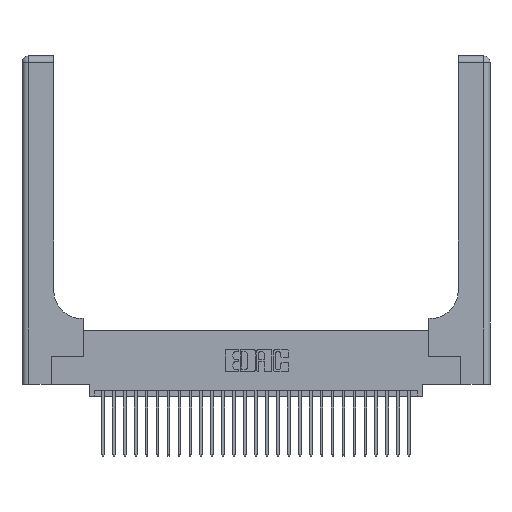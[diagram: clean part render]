
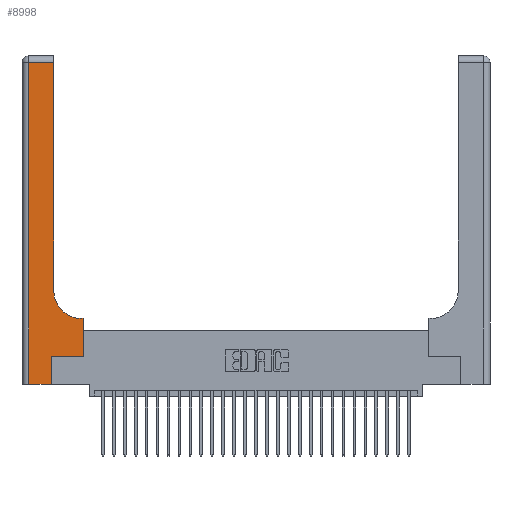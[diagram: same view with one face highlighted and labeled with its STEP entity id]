
A CAD part, top view. The second image highlights one B-rep face of the part: STEP entity #8998.
In plain terms, the highlighted planar face has unit normal (0, 0, 1).
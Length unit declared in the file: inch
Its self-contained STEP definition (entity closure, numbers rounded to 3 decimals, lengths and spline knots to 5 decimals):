
#754 = EDGE_CURVE ( 'NONE', #13265, #20896, #26308, .T. ) ;
#1070 = CIRCLE ( 'NONE', #4278, 0.25 ) ;
#1675 = EDGE_CURVE ( 'NONE', #7780, #22664, #6212, .T. ) ;
#1995 = CARTESIAN_POINT ( 'NONE',  ( 0., 2.94, 0.37 ) ) ;
#3305 = CARTESIAN_POINT ( 'NONE',  ( 0.5585, 0.25, 0.37 ) ) ;
#3576 = VERTEX_POINT ( 'NONE', #15224 ) ;
#3621 = DIRECTION ( 'NONE',  ( 0., 0., -1. ) ) ;
#3798 = CARTESIAN_POINT ( 'NONE',  ( 0.269, 0.25, 0.37 ) ) ;
#3932 = CARTESIAN_POINT ( 'NONE',  ( 0.5585, 0.6, 0.37 ) ) ;
#4256 = ORIENTED_EDGE ( 'NONE', *, *, #15265, .T. ) ;
#4278 = AXIS2_PLACEMENT_3D ( 'NONE', #15434, #3621, #26717 ) ;
#4520 = ORIENTED_EDGE ( 'NONE', *, *, #28610, .T. ) ;
#4866 = CARTESIAN_POINT ( 'NONE',  ( 0., 0., 0.37 ) ) ;
#5934 = DIRECTION ( 'NONE',  ( 1., 0., 0. ) ) ;
#6010 = FACE_OUTER_BOUND ( 'NONE', #8364, .T. ) ;
#6212 = LINE ( 'NONE', #3305, #18464 ) ;
#6389 = DIRECTION ( 'NONE',  ( 0., -1., 0. ) ) ;
#6430 = LINE ( 'NONE', #4866, #6605 ) ;
#6605 = VECTOR ( 'NONE', #23003, 39.37008 ) ;
#6891 = PLANE ( 'NONE',  #25453 ) ;
#6987 = CARTESIAN_POINT ( 'NONE',  ( 0., 3., 0.37 ) ) ;
#7747 = ORIENTED_EDGE ( 'NONE', *, *, #21952, .T. ) ;
#7780 = VERTEX_POINT ( 'NONE', #9403 ) ;
#8282 = VECTOR ( 'NONE', #20850, 39.37008 ) ;
#8323 = ORIENTED_EDGE ( 'NONE', *, *, #13071, .T. ) ;
#8364 = EDGE_LOOP ( 'NONE', ( #8323, #23698, #21033, #4256, #4520, #16832, #18394, #7747, #14993 ) ) ;
#8381 = LINE ( 'NONE', #16897, #18466 ) ;
#8575 = VERTEX_POINT ( 'NONE', #25861 ) ;
#8998 = ADVANCED_FACE ( 'NONE', ( #6010 ), #6891, .F. ) ;
#9403 = CARTESIAN_POINT ( 'NONE',  ( 0.5585, 0.25, 0.37 ) ) ;
#9794 = LINE ( 'NONE', #24581, #23461 ) ;
#11615 = CARTESIAN_POINT ( 'NONE',  ( 0.269, 0., 0.37 ) ) ;
#11818 = VERTEX_POINT ( 'NONE', #25079 ) ;
#12091 = DIRECTION ( 'NONE',  ( -1., 0., 0. ) ) ;
#12625 = LINE ( 'NONE', #11615, #8282 ) ;
#13071 = EDGE_CURVE ( 'NONE', #29853, #13265, #13387, .T. ) ;
#13265 = VERTEX_POINT ( 'NONE', #22595 ) ;
#13387 = LINE ( 'NONE', #17493, #26680 ) ;
#13688 = CARTESIAN_POINT ( 'NONE',  ( 0.269, 0.25, 0.37 ) ) ;
#14337 = EDGE_CURVE ( 'NONE', #16971, #7780, #27714, .T. ) ;
#14993 = ORIENTED_EDGE ( 'NONE', *, *, #22571, .T. ) ;
#15101 = CARTESIAN_POINT ( 'NONE',  ( 0.06, 2.94, 0.37 ) ) ;
#15103 = VECTOR ( 'NONE', #5934, 39.37008 ) ;
#15224 = CARTESIAN_POINT ( 'NONE',  ( 0.5415, 0.6, 0.37 ) ) ;
#15254 = CARTESIAN_POINT ( 'NONE',  ( 0.2915, 0.85, 0.37 ) ) ;
#15265 = EDGE_CURVE ( 'NONE', #8575, #11818, #6430, .T. ) ;
#15434 = CARTESIAN_POINT ( 'NONE',  ( 0.5415, 0.85, 0.37 ) ) ;
#16832 = ORIENTED_EDGE ( 'NONE', *, *, #14337, .T. ) ;
#16897 = CARTESIAN_POINT ( 'NONE',  ( 0.2915, 0.6, 0.37 ) ) ;
#16971 = VERTEX_POINT ( 'NONE', #13688 ) ;
#17493 = CARTESIAN_POINT ( 'NONE',  ( 0.2915, 3., 0.37 ) ) ;
#18394 = ORIENTED_EDGE ( 'NONE', *, *, #1675, .T. ) ;
#18464 = VECTOR ( 'NONE', #21605, 39.37008 ) ;
#18466 = VECTOR ( 'NONE', #12091, 39.37008 ) ;
#18537 = EDGE_CURVE ( 'NONE', #20896, #8575, #9794, .T. ) ;
#20193 = VECTOR ( 'NONE', #22867, 39.37008 ) ;
#20850 = DIRECTION ( 'NONE',  ( 0., 1., 0. ) ) ;
#20896 = VERTEX_POINT ( 'NONE', #15101 ) ;
#21033 = ORIENTED_EDGE ( 'NONE', *, *, #18537, .T. ) ;
#21605 = DIRECTION ( 'NONE',  ( 0., 1., 0. ) ) ;
#21952 = EDGE_CURVE ( 'NONE', #22664, #3576, #8381, .T. ) ;
#22571 = EDGE_CURVE ( 'NONE', #3576, #29853, #1070, .T. ) ;
#22595 = CARTESIAN_POINT ( 'NONE',  ( 0.2915, 2.94, 0.37 ) ) ;
#22664 = VERTEX_POINT ( 'NONE', #3932 ) ;
#22867 = DIRECTION ( 'NONE',  ( -1., 0., 0. ) ) ;
#22878 = DIRECTION ( 'NONE',  ( -1., 0., 0. ) ) ;
#22979 = DIRECTION ( 'NONE',  ( 0., 0., -1. ) ) ;
#23003 = DIRECTION ( 'NONE',  ( 1., 0., 0. ) ) ;
#23461 = VECTOR ( 'NONE', #6389, 39.37008 ) ;
#23698 = ORIENTED_EDGE ( 'NONE', *, *, #754, .T. ) ;
#24581 = CARTESIAN_POINT ( 'NONE',  ( 0.06, 3., 0.37 ) ) ;
#25079 = CARTESIAN_POINT ( 'NONE',  ( 0.269, 0., 0.37 ) ) ;
#25453 = AXIS2_PLACEMENT_3D ( 'NONE', #6987, #22979, #22878 ) ;
#25861 = CARTESIAN_POINT ( 'NONE',  ( 0.06, 0., 0.37 ) ) ;
#26308 = LINE ( 'NONE', #1995, #20193 ) ;
#26680 = VECTOR ( 'NONE', #28956, 39.37008 ) ;
#26717 = DIRECTION ( 'NONE',  ( 1., 0., 0. ) ) ;
#27714 = LINE ( 'NONE', #3798, #15103 ) ;
#28610 = EDGE_CURVE ( 'NONE', #11818, #16971, #12625, .T. ) ;
#28956 = DIRECTION ( 'NONE',  ( 0., 1., 0. ) ) ;
#29853 = VERTEX_POINT ( 'NONE', #15254 ) ;
